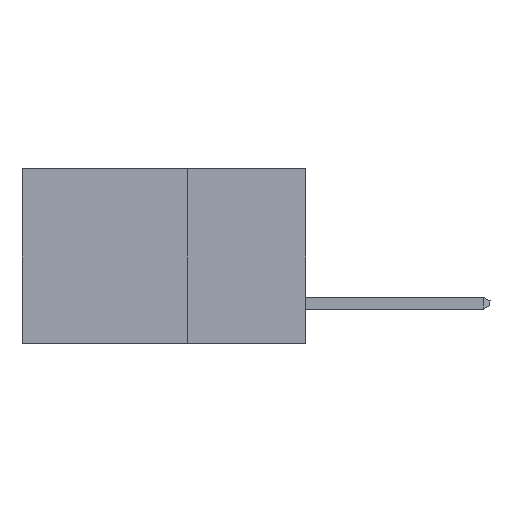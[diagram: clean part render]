
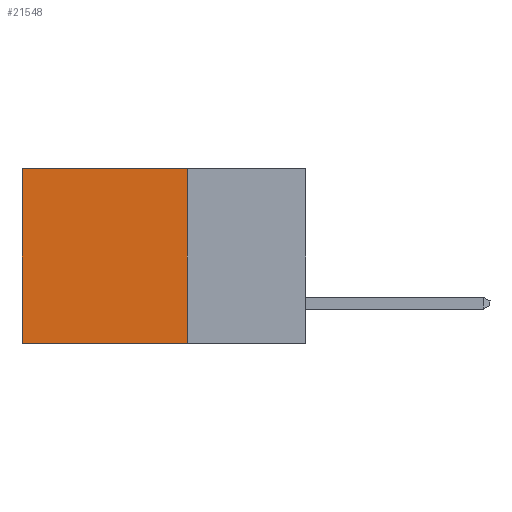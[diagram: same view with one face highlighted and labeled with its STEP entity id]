
A CAD part, left-side view. The second image highlights one B-rep face of the part: STEP entity #21548.
In plain terms, the highlighted planar face has unit normal (-1, 0, 0).
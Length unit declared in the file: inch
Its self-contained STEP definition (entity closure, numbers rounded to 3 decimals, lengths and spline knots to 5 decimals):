
#929 = DIRECTION ( 'NONE',  ( 0., 0., -1. ) ) ;
#963 = DIRECTION ( 'NONE',  ( 0., 1., 0. ) ) ;
#1575 = VERTEX_POINT ( 'NONE', #16361 ) ;
#2405 = EDGE_CURVE ( 'NONE', #14623, #18758, #8994, .T. ) ;
#2448 = LINE ( 'NONE', #10231, #11310 ) ;
#4000 = EDGE_CURVE ( 'NONE', #19624, #1575, #12273, .T. ) ;
#4373 = CARTESIAN_POINT ( 'NONE',  ( 0.2615, 0.25, -0.37 ) ) ;
#4459 = LINE ( 'NONE', #12621, #24408 ) ;
#6047 = DIRECTION ( 'NONE',  ( 0., 1., 0. ) ) ;
#8560 = VECTOR ( 'NONE', #963, 39.37008 ) ;
#8994 = LINE ( 'NONE', #24479, #8560 ) ;
#9196 = DIRECTION ( 'NONE',  ( 0., 0., -1. ) ) ;
#10231 = CARTESIAN_POINT ( 'NONE',  ( 0.2615, 0.25, -0.37 ) ) ;
#10814 = ORIENTED_EDGE ( 'NONE', *, *, #17174, .F. ) ;
#10872 = AXIS2_PLACEMENT_3D ( 'NONE', #18757, #13142, #9196 ) ;
#11310 = VECTOR ( 'NONE', #929, 39.37008 ) ;
#12061 = ORIENTED_EDGE ( 'NONE', *, *, #19571, .T. ) ;
#12273 = LINE ( 'NONE', #4373, #22561 ) ;
#12303 = ORIENTED_EDGE ( 'NONE', *, *, #2405, .T. ) ;
#12621 = CARTESIAN_POINT ( 'NONE',  ( 0.2615, 0.6, -0.37 ) ) ;
#13142 = DIRECTION ( 'NONE',  ( 1., 0., 0. ) ) ;
#13181 = CARTESIAN_POINT ( 'NONE',  ( 0.2615, 0.6, 0. ) ) ;
#14289 = DIRECTION ( 'NONE',  ( 0., 0., -1. ) ) ;
#14623 = VERTEX_POINT ( 'NONE', #23519 ) ;
#14786 = CARTESIAN_POINT ( 'NONE',  ( 0.2615, 0.25, -0.37 ) ) ;
#15458 = FACE_OUTER_BOUND ( 'NONE', #23727, .T. ) ;
#16361 = CARTESIAN_POINT ( 'NONE',  ( 0.2615, 0.6, -0.37 ) ) ;
#17174 = EDGE_CURVE ( 'NONE', #14623, #19624, #2448, .T. ) ;
#18757 = CARTESIAN_POINT ( 'NONE',  ( 0.2615, 0.25, -0.37 ) ) ;
#18758 = VERTEX_POINT ( 'NONE', #13181 ) ;
#19143 = PLANE ( 'NONE',  #10872 ) ;
#19571 = EDGE_CURVE ( 'NONE', #18758, #1575, #4459, .T. ) ;
#19624 = VERTEX_POINT ( 'NONE', #14786 ) ;
#21102 = ORIENTED_EDGE ( 'NONE', *, *, #4000, .F. ) ;
#21548 = ADVANCED_FACE ( 'NONE', ( #15458 ), #19143, .F. ) ;
#22561 = VECTOR ( 'NONE', #6047, 39.37008 ) ;
#23519 = CARTESIAN_POINT ( 'NONE',  ( 0.2615, 0.25, 0. ) ) ;
#23727 = EDGE_LOOP ( 'NONE', ( #12061, #21102, #10814, #12303 ) ) ;
#24408 = VECTOR ( 'NONE', #14289, 39.37008 ) ;
#24479 = CARTESIAN_POINT ( 'NONE',  ( 0.2615, 0.25, 0. ) ) ;
